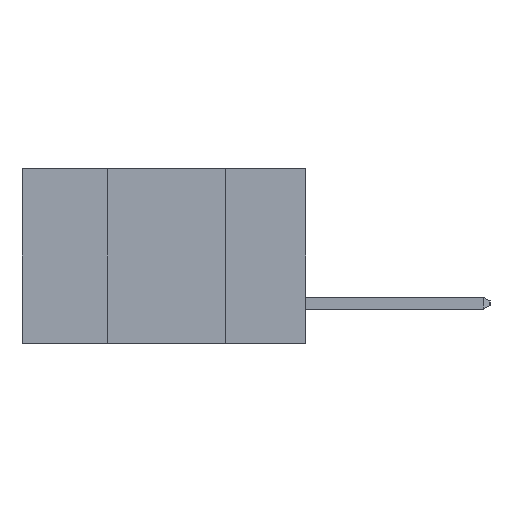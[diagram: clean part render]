
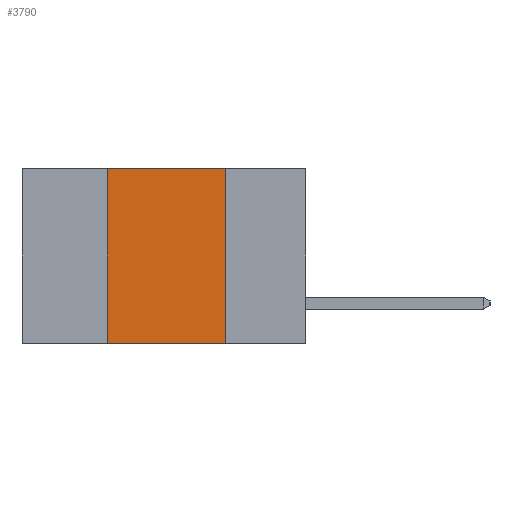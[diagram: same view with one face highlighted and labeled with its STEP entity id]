
A CAD part, left-side view. The second image highlights one B-rep face of the part: STEP entity #3790.
In plain terms, the highlighted planar face has unit normal (-1, 0, 0).
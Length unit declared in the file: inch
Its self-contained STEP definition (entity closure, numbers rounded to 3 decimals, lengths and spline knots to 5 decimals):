
#170 = CARTESIAN_POINT ( 'NONE',  ( 0., 0.17, 0. ) ) ;
#293 = EDGE_CURVE ( 'NONE', #12226, #7965, #9170, .T. ) ;
#884 = AXIS2_PLACEMENT_3D ( 'NONE', #1773, #1460, #1431 ) ;
#964 = EDGE_CURVE ( 'NONE', #4494, #12226, #3907, .T. ) ;
#1037 = CARTESIAN_POINT ( 'NONE',  ( 0., 0.42, 0. ) ) ;
#1252 = ORIENTED_EDGE ( 'NONE', *, *, #8464, .T. ) ;
#1431 = DIRECTION ( 'NONE',  ( 0., 0., -1. ) ) ;
#1460 = DIRECTION ( 'NONE',  ( 1., 0., 0. ) ) ;
#1464 = PLANE ( 'NONE',  #884 ) ;
#1710 = LINE ( 'NONE', #2920, #10983 ) ;
#1773 = CARTESIAN_POINT ( 'NONE',  ( 0., 0.6, 0. ) ) ;
#2142 = DIRECTION ( 'NONE',  ( 0., 0., 1. ) ) ;
#2920 = CARTESIAN_POINT ( 'NONE',  ( 0., 0.6, -0.37 ) ) ;
#3213 = ORIENTED_EDGE ( 'NONE', *, *, #964, .F. ) ;
#3569 = VECTOR ( 'NONE', #13514, 39.37008 ) ;
#3790 = ADVANCED_FACE ( 'NONE', ( #13875 ), #1464, .F. ) ;
#3907 = LINE ( 'NONE', #14157, #3569 ) ;
#4038 = DIRECTION ( 'NONE',  ( 0., -1., 0. ) ) ;
#4494 = VERTEX_POINT ( 'NONE', #1037 ) ;
#6169 = VECTOR ( 'NONE', #11315, 39.37008 ) ;
#6236 = VERTEX_POINT ( 'NONE', #10440 ) ;
#7656 = CARTESIAN_POINT ( 'NONE',  ( 0., 0.17, -0.37 ) ) ;
#7965 = VERTEX_POINT ( 'NONE', #7656 ) ;
#8464 = EDGE_CURVE ( 'NONE', #6236, #7965, #1710, .T. ) ;
#8576 = LINE ( 'NONE', #9940, #14087 ) ;
#9105 = EDGE_CURVE ( 'NONE', #6236, #4494, #8576, .T. ) ;
#9170 = LINE ( 'NONE', #12583, #6169 ) ;
#9749 = ORIENTED_EDGE ( 'NONE', *, *, #9105, .F. ) ;
#9940 = CARTESIAN_POINT ( 'NONE',  ( 0., 0.42, -0.37 ) ) ;
#10150 = EDGE_LOOP ( 'NONE', ( #11142, #3213, #9749, #1252 ) ) ;
#10440 = CARTESIAN_POINT ( 'NONE',  ( 0., 0.42, -0.37 ) ) ;
#10983 = VECTOR ( 'NONE', #4038, 39.37008 ) ;
#11142 = ORIENTED_EDGE ( 'NONE', *, *, #293, .F. ) ;
#11315 = DIRECTION ( 'NONE',  ( 0., 0., -1. ) ) ;
#12226 = VERTEX_POINT ( 'NONE', #170 ) ;
#12583 = CARTESIAN_POINT ( 'NONE',  ( 0., 0.17, -0.37 ) ) ;
#13514 = DIRECTION ( 'NONE',  ( 0., -1., 0. ) ) ;
#13875 = FACE_OUTER_BOUND ( 'NONE', #10150, .T. ) ;
#14087 = VECTOR ( 'NONE', #2142, 39.37008 ) ;
#14157 = CARTESIAN_POINT ( 'NONE',  ( 0., 0.6, 0. ) ) ;
